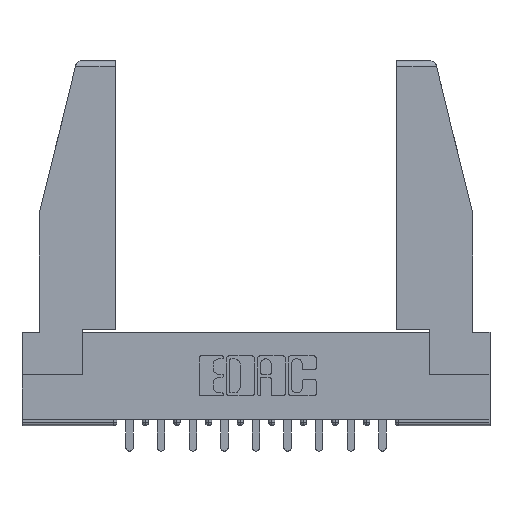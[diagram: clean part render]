
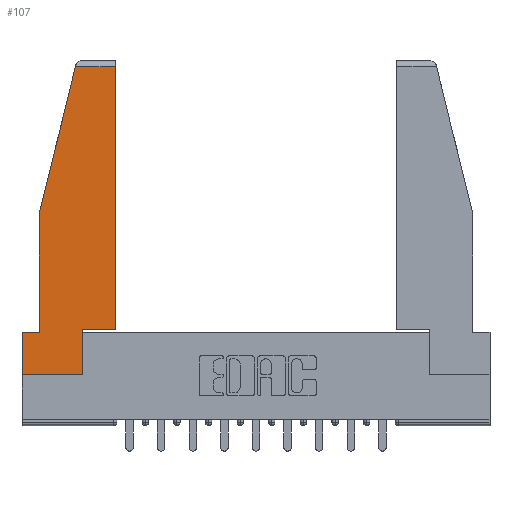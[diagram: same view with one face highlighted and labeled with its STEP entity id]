
A CAD part, top view. The second image highlights one B-rep face of the part: STEP entity #107.
In plain terms, the highlighted planar face has unit normal (0, 0, 1).
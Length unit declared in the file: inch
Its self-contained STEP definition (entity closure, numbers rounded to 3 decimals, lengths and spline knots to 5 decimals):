
#107 = ADVANCED_FACE ( 'NONE', ( #8502 ), #12140, .T. ) ;
#154 = DIRECTION ( 'NONE',  ( 0., -1., 0. ) ) ;
#253 = EDGE_LOOP ( 'NONE', ( #8093, #8399, #12586, #13139, #5524, #14416, #4223, #2021, #13380 ) ) ;
#326 = CARTESIAN_POINT ( 'NONE',  ( 0.086, 0.8, 0. ) ) ;
#649 = VECTOR ( 'NONE', #9857, 39.37008 ) ;
#978 = CARTESIAN_POINT ( 'NONE',  ( 0.086, 0.21, 0. ) ) ;
#995 = CARTESIAN_POINT ( 'NONE',  ( 0.086, 0.8, 0. ) ) ;
#1518 = CARTESIAN_POINT ( 'NONE',  ( 0.461, 1.52, 0. ) ) ;
#1707 = EDGE_CURVE ( 'NONE', #12225, #9130, #9393, .T. ) ;
#1760 = EDGE_CURVE ( 'NONE', #2945, #13943, #2159, .T. ) ;
#1823 = VECTOR ( 'NONE', #12047, 39.37008 ) ;
#2021 = ORIENTED_EDGE ( 'NONE', *, *, #14841, .T. ) ;
#2148 = CARTESIAN_POINT ( 'NONE',  ( 0., 0.21, 0. ) ) ;
#2159 = LINE ( 'NONE', #5661, #7216 ) ;
#2225 = DIRECTION ( 'NONE',  ( -0.239, -0.971, 0. ) ) ;
#2483 = CARTESIAN_POINT ( 'NONE',  ( 0.461, 0.223, 0. ) ) ;
#2945 = VERTEX_POINT ( 'NONE', #2148 ) ;
#3381 = VERTEX_POINT ( 'NONE', #2483 ) ;
#3474 = VERTEX_POINT ( 'NONE', #5081 ) ;
#3520 = EDGE_CURVE ( 'NONE', #9130, #10768, #6380, .T. ) ;
#3747 = CARTESIAN_POINT ( 'NONE',  ( 0., 1.52, 0. ) ) ;
#3913 = EDGE_CURVE ( 'NONE', #9253, #12225, #10755, .T. ) ;
#4052 = CARTESIAN_POINT ( 'NONE',  ( 0., 0., 0. ) ) ;
#4223 = ORIENTED_EDGE ( 'NONE', *, *, #7053, .T. ) ;
#5081 = CARTESIAN_POINT ( 'NONE',  ( 0.297, 0.223, 0. ) ) ;
#5129 = DIRECTION ( 'NONE',  ( 0., 1., 0. ) ) ;
#5140 = CARTESIAN_POINT ( 'NONE',  ( 0., 0., 0. ) ) ;
#5160 = CARTESIAN_POINT ( 'NONE',  ( 0., 0., 0. ) ) ;
#5524 = ORIENTED_EDGE ( 'NONE', *, *, #13416, .T. ) ;
#5555 = EDGE_CURVE ( 'NONE', #3474, #3381, #14339, .T. ) ;
#5661 = CARTESIAN_POINT ( 'NONE',  ( 0., 0.21, 0. ) ) ;
#5969 = VECTOR ( 'NONE', #7600, 39.37008 ) ;
#6054 = VECTOR ( 'NONE', #12322, 39.37008 ) ;
#6179 = CARTESIAN_POINT ( 'NONE',  ( 0.297, 0.223, 0. ) ) ;
#6380 = LINE ( 'NONE', #326, #10408 ) ;
#6411 = CARTESIAN_POINT ( 'NONE',  ( 0.297, 0., 0. ) ) ;
#6523 = LINE ( 'NONE', #5140, #5969 ) ;
#6816 = VECTOR ( 'NONE', #10364, 39.37008 ) ;
#6969 = CARTESIAN_POINT ( 'NONE',  ( 0.271, 1.55, 0. ) ) ;
#7053 = EDGE_CURVE ( 'NONE', #13943, #9498, #6523, .T. ) ;
#7105 = CARTESIAN_POINT ( 'NONE',  ( 0., 0.21, 0. ) ) ;
#7171 = AXIS2_PLACEMENT_3D ( 'NONE', #4052, #13359, #9700 ) ;
#7216 = VECTOR ( 'NONE', #154, 39.37008 ) ;
#7600 = DIRECTION ( 'NONE',  ( 1., 0., 0. ) ) ;
#8093 = ORIENTED_EDGE ( 'NONE', *, *, #12863, .T. ) ;
#8248 = LINE ( 'NONE', #7105, #6816 ) ;
#8399 = ORIENTED_EDGE ( 'NONE', *, *, #3913, .T. ) ;
#8502 = FACE_OUTER_BOUND ( 'NONE', #253, .T. ) ;
#8584 = CARTESIAN_POINT ( 'NONE',  ( 0.297, 0., 0. ) ) ;
#8769 = LINE ( 'NONE', #13553, #6054 ) ;
#9130 = VERTEX_POINT ( 'NONE', #995 ) ;
#9253 = VERTEX_POINT ( 'NONE', #1518 ) ;
#9393 = LINE ( 'NONE', #6969, #13037 ) ;
#9498 = VERTEX_POINT ( 'NONE', #6411 ) ;
#9700 = DIRECTION ( 'NONE',  ( 1., 0., 0. ) ) ;
#9857 = DIRECTION ( 'NONE',  ( -1., 0., 0. ) ) ;
#9962 = DIRECTION ( 'NONE',  ( 0., -1., 0. ) ) ;
#10364 = DIRECTION ( 'NONE',  ( -1., 0., 0. ) ) ;
#10408 = VECTOR ( 'NONE', #9962, 39.37008 ) ;
#10755 = LINE ( 'NONE', #3747, #649 ) ;
#10768 = VERTEX_POINT ( 'NONE', #978 ) ;
#11675 = CARTESIAN_POINT ( 'NONE',  ( 0.2636, 1.52, 0. ) ) ;
#11764 = LINE ( 'NONE', #8584, #13039 ) ;
#12047 = DIRECTION ( 'NONE',  ( 1., 0., 0. ) ) ;
#12140 = PLANE ( 'NONE',  #7171 ) ;
#12225 = VERTEX_POINT ( 'NONE', #11675 ) ;
#12322 = DIRECTION ( 'NONE',  ( 0., 1., 0. ) ) ;
#12586 = ORIENTED_EDGE ( 'NONE', *, *, #1707, .T. ) ;
#12863 = EDGE_CURVE ( 'NONE', #3381, #9253, #8769, .T. ) ;
#13037 = VECTOR ( 'NONE', #2225, 39.37008 ) ;
#13039 = VECTOR ( 'NONE', #5129, 39.37008 ) ;
#13139 = ORIENTED_EDGE ( 'NONE', *, *, #3520, .T. ) ;
#13359 = DIRECTION ( 'NONE',  ( 0., 0., 1. ) ) ;
#13380 = ORIENTED_EDGE ( 'NONE', *, *, #5555, .T. ) ;
#13416 = EDGE_CURVE ( 'NONE', #10768, #2945, #8248, .T. ) ;
#13553 = CARTESIAN_POINT ( 'NONE',  ( 0.461, 0.223, 0. ) ) ;
#13943 = VERTEX_POINT ( 'NONE', #5160 ) ;
#14339 = LINE ( 'NONE', #6179, #1823 ) ;
#14416 = ORIENTED_EDGE ( 'NONE', *, *, #1760, .T. ) ;
#14841 = EDGE_CURVE ( 'NONE', #9498, #3474, #11764, .T. ) ;
